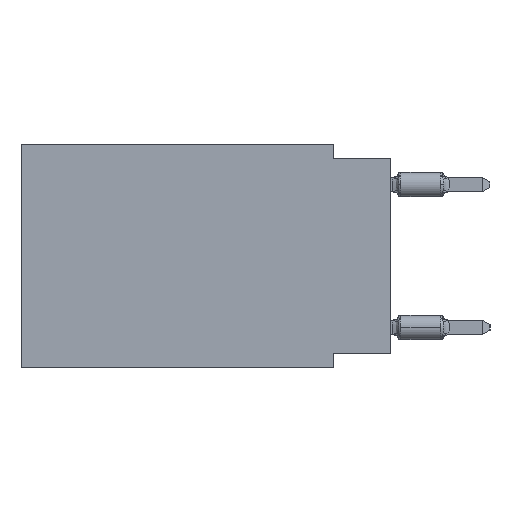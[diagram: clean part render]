
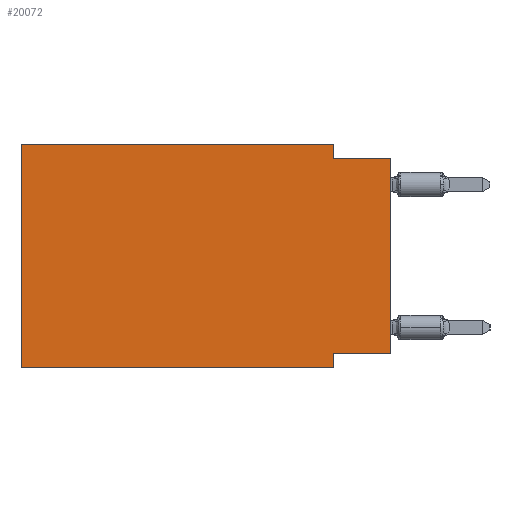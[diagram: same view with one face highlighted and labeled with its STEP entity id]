
A CAD part, left-side view. The second image highlights one B-rep face of the part: STEP entity #20072.
In plain terms, the highlighted planar face has unit normal (-1, 0, 0).
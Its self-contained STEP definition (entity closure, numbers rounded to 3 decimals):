
#287 = CARTESIAN_POINT ( 'NONE',  ( 0., 2.54, -9.906 ) ) ;
#502 = VECTOR ( 'NONE', #7428, 1000. ) ;
#839 = VECTOR ( 'NONE', #26601, 1000. ) ;
#939 = CARTESIAN_POINT ( 'NONE',  ( 0., 2.54, 0. ) ) ;
#1237 = VERTEX_POINT ( 'NONE', #10836 ) ;
#2271 = VERTEX_POINT ( 'NONE', #6291 ) ;
#2484 = LINE ( 'NONE', #12516, #29312 ) ;
#2561 = PLANE ( 'NONE',  #16835 ) ;
#2772 = DIRECTION ( 'NONE',  ( 0., 1., 0. ) ) ;
#2785 = CARTESIAN_POINT ( 'NONE',  ( 0., 2.54, 0. ) ) ;
#2847 = ORIENTED_EDGE ( 'NONE', *, *, #16816, .T. ) ;
#3724 = EDGE_LOOP ( 'NONE', ( #2847, #5284, #25379, #32037, #12911, #27051, #14342, #15569 ) ) ;
#5094 = VECTOR ( 'NONE', #15127, 1000. ) ;
#5284 = ORIENTED_EDGE ( 'NONE', *, *, #27537, .F. ) ;
#5309 = CARTESIAN_POINT ( 'NONE',  ( 0., 2.54, -0.635 ) ) ;
#5473 = CARTESIAN_POINT ( 'NONE',  ( 0., 0., -0.635 ) ) ;
#6291 = CARTESIAN_POINT ( 'NONE',  ( 0., 0., -9.271 ) ) ;
#6783 = EDGE_CURVE ( 'NONE', #2271, #1237, #14785, .T. ) ;
#7379 = LINE ( 'NONE', #17447, #5094 ) ;
#7428 = DIRECTION ( 'NONE',  ( 0., -1., 0. ) ) ;
#7924 = VECTOR ( 'NONE', #11299, 1000. ) ;
#8026 = EDGE_CURVE ( 'NONE', #1237, #11432, #30450, .T. ) ;
#9240 = CARTESIAN_POINT ( 'NONE',  ( 0., 0., -0.635 ) ) ;
#9943 = CARTESIAN_POINT ( 'NONE',  ( 0., 16.383, -9.906 ) ) ;
#10836 = CARTESIAN_POINT ( 'NONE',  ( 0., 2.54, -9.271 ) ) ;
#11299 = DIRECTION ( 'NONE',  ( 0., 0., -1. ) ) ;
#11379 = EDGE_CURVE ( 'NONE', #25055, #30721, #2484, .T. ) ;
#11432 = VERTEX_POINT ( 'NONE', #30336 ) ;
#11985 = CARTESIAN_POINT ( 'NONE',  ( 0., 16.383, 0. ) ) ;
#12370 = CARTESIAN_POINT ( 'NONE',  ( 0., 16.383, 0. ) ) ;
#12516 = CARTESIAN_POINT ( 'NONE',  ( 0., 16.383, 0. ) ) ;
#12597 = DIRECTION ( 'NONE',  ( 0., 0., -1. ) ) ;
#12768 = DIRECTION ( 'NONE',  ( 1., 0., 0. ) ) ;
#12841 = LINE ( 'NONE', #939, #7924 ) ;
#12911 = ORIENTED_EDGE ( 'NONE', *, *, #11379, .F. ) ;
#12953 = DIRECTION ( 'NONE',  ( 0., 0., -1. ) ) ;
#14342 = ORIENTED_EDGE ( 'NONE', *, *, #8026, .F. ) ;
#14767 = VERTEX_POINT ( 'NONE', #5473 ) ;
#14785 = LINE ( 'NONE', #27329, #26291 ) ;
#15127 = DIRECTION ( 'NONE',  ( 0., 0., 1. ) ) ;
#15409 = DIRECTION ( 'NONE',  ( 0., -1., 0. ) ) ;
#15569 = ORIENTED_EDGE ( 'NONE', *, *, #6783, .F. ) ;
#16816 = EDGE_CURVE ( 'NONE', #2271, #14767, #7379, .T. ) ;
#16835 = AXIS2_PLACEMENT_3D ( 'NONE', #32555, #12768, #12597 ) ;
#17447 = CARTESIAN_POINT ( 'NONE',  ( 0., 0., 0. ) ) ;
#17598 = EDGE_CURVE ( 'NONE', #30721, #29687, #22274, .T. ) ;
#19990 = VECTOR ( 'NONE', #15409, 1000. ) ;
#20071 = EDGE_CURVE ( 'NONE', #25055, #11432, #22485, .T. ) ;
#20072 = ADVANCED_FACE ( 'NONE', ( #29927 ), #2561, .F. ) ;
#21055 = EDGE_CURVE ( 'NONE', #29687, #24569, #12841, .T. ) ;
#22274 = LINE ( 'NONE', #12370, #502 ) ;
#22485 = LINE ( 'NONE', #9943, #19990 ) ;
#22900 = CARTESIAN_POINT ( 'NONE',  ( 0., 16.383, -9.906 ) ) ;
#24569 = VERTEX_POINT ( 'NONE', #5309 ) ;
#25055 = VERTEX_POINT ( 'NONE', #22900 ) ;
#25379 = ORIENTED_EDGE ( 'NONE', *, *, #21055, .F. ) ;
#26291 = VECTOR ( 'NONE', #2772, 1000. ) ;
#26601 = DIRECTION ( 'NONE',  ( 0., -1., 0. ) ) ;
#27051 = ORIENTED_EDGE ( 'NONE', *, *, #20071, .T. ) ;
#27329 = CARTESIAN_POINT ( 'NONE',  ( 0., 0., -9.271 ) ) ;
#27537 = EDGE_CURVE ( 'NONE', #24569, #14767, #29090, .T. ) ;
#29090 = LINE ( 'NONE', #9240, #839 ) ;
#29312 = VECTOR ( 'NONE', #31406, 1000. ) ;
#29687 = VERTEX_POINT ( 'NONE', #2785 ) ;
#29927 = FACE_OUTER_BOUND ( 'NONE', #3724, .T. ) ;
#30336 = CARTESIAN_POINT ( 'NONE',  ( 0., 2.54, -9.906 ) ) ;
#30450 = LINE ( 'NONE', #287, #31064 ) ;
#30721 = VERTEX_POINT ( 'NONE', #11985 ) ;
#31064 = VECTOR ( 'NONE', #12953, 1000. ) ;
#31406 = DIRECTION ( 'NONE',  ( 0., 0., 1. ) ) ;
#32037 = ORIENTED_EDGE ( 'NONE', *, *, #17598, .F. ) ;
#32555 = CARTESIAN_POINT ( 'NONE',  ( 0., 16.383, 0. ) ) ;
